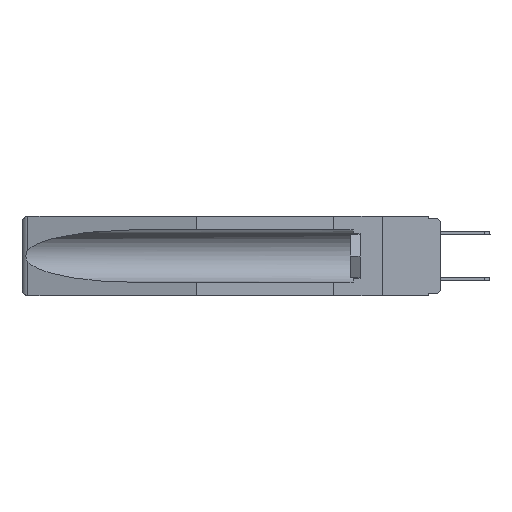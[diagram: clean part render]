
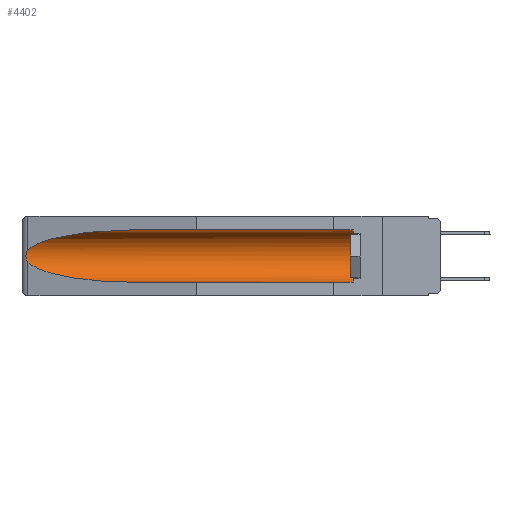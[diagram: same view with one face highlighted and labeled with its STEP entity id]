
A CAD part, left-side view. The second image highlights one B-rep face of the part: STEP entity #4402.
In plain terms, the highlighted cylindrical face has radius 2.857 mm (diameter 5.715 mm), a partial arc.
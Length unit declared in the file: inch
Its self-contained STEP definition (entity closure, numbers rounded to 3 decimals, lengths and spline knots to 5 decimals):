
#233 = CARTESIAN_POINT ( 'NONE',  ( 0.2675, 1.53308, -0.16763 ) ) ;
#564 = CARTESIAN_POINT ( 'NONE',  ( 0.21114, 1.30732, -0.059 ) ) ;
#1021 = CARTESIAN_POINT ( 'NONE',  ( 0.155, 1.07973, -0.284 ) ) ;
#1022 = ORIENTED_EDGE ( 'NONE', *, *, #17976, .T. ) ;
#1430 = LINE ( 'NONE', #1641, #16844 ) ;
#1641 = CARTESIAN_POINT ( 'NONE',  ( 0.155, -0.30754, -0.059 ) ) ;
#2132 = CARTESIAN_POINT ( 'NONE',  ( 0.155, 1.07973, -0.059 ) ) ;
#2237 = CARTESIAN_POINT ( 'NONE',  ( 0.25451, 1.48313, -0.09465 ) ) ;
#2512 = CARTESIAN_POINT ( 'NONE',  ( 0.155, 0.126, -0.059 ) ) ;
#2691 = FACE_OUTER_BOUND ( 'NONE', #11724, .T. ) ;
#2949 = CARTESIAN_POINT ( 'NONE',  ( 0.26597, 1.5296, -0.19026 ) ) ;
#3265 = CARTESIAN_POINT ( 'NONE',  ( 0.26537, 1.52718, -0.19328 ) ) ;
#3287 =( BOUNDED_CURVE ( )  B_SPLINE_CURVE ( 3, ( #2132, #564, #2237, #11764 ),
 .UNSPECIFIED., .F., .F. ) 
 B_SPLINE_CURVE_WITH_KNOTS ( ( 4, 4 ),
 ( 4.71239, 6.08839 ),
 .UNSPECIFIED. ) 
 CURVE ( )  GEOMETRIC_REPRESENTATION_ITEM ( )  RATIONAL_B_SPLINE_CURVE ( ( 1., 0.848, 0.848, 1. ) ) 
 REPRESENTATION_ITEM ( '' )  );
#4231 = VERTEX_POINT ( 'NONE', #16061 ) ;
#4356 = CARTESIAN_POINT ( 'NONE',  ( 0.25451, 1.48313, -0.24835 ) ) ;
#4402 = ADVANCED_FACE ( 'NONE', ( #2691 ), #16891, .F. ) ;
#4617 = CARTESIAN_POINT ( 'NONE',  ( 0.26655, 1.53094, -0.18657 ) ) ;
#4710 = CARTESIAN_POINT ( 'NONE',  ( 0.155, 1.07973, -0.284 ) ) ;
#4714 = CARTESIAN_POINT ( 'NONE',  ( 0.2673, 1.5327, -0.16383 ) ) ;
#5060 = ORIENTED_EDGE ( 'NONE', *, *, #8075, .T. ) ;
#5434 = ORIENTED_EDGE ( 'NONE', *, *, #13856, .T. ) ;
#5784 = CARTESIAN_POINT ( 'NONE',  ( 0.155, 0.126, -0.1715 ) ) ;
#6105 = VERTEX_POINT ( 'NONE', #10106 ) ;
#6352 = DIRECTION ( 'NONE',  ( 0., 1., 0. ) ) ;
#6430 = EDGE_CURVE ( 'NONE', #4231, #14896, #3287, .T. ) ;
#6797 = VERTEX_POINT ( 'NONE', #4710 ) ;
#7406 = DIRECTION ( 'NONE',  ( 0., 0., 1. ) ) ;
#8075 = EDGE_CURVE ( 'NONE', #14896, #6105, #18001, .T. ) ;
#8991 = CARTESIAN_POINT ( 'NONE',  ( 0.26537, 1.52718, -0.19328 ) ) ;
#9757 = CARTESIAN_POINT ( 'NONE',  ( 0.26537, 1.52718, -0.14972 ) ) ;
#9837 = ORIENTED_EDGE ( 'NONE', *, *, #15419, .F. ) ;
#10106 = CARTESIAN_POINT ( 'NONE',  ( 0.26537, 1.52718, -0.19328 ) ) ;
#10739 = CARTESIAN_POINT ( 'NONE',  ( 0.21114, 1.30732, -0.284 ) ) ;
#11294 = VERTEX_POINT ( 'NONE', #11916 ) ;
#11454 = CARTESIAN_POINT ( 'NONE',  ( 0.155, -0.30754, -0.284 ) ) ;
#11478 = VECTOR ( 'NONE', #11559, 39.37008 ) ;
#11559 = DIRECTION ( 'NONE',  ( 0., 1., 0. ) ) ;
#11724 = EDGE_LOOP ( 'NONE', ( #20489, #5060, #5434, #9837, #19543, #1022 ) ) ;
#11764 = CARTESIAN_POINT ( 'NONE',  ( 0.26537, 1.52718, -0.14972 ) ) ;
#11916 = CARTESIAN_POINT ( 'NONE',  ( 0.155, 0.126, -0.284 ) ) ;
#12259 = AXIS2_PLACEMENT_3D ( 'NONE', #17091, #15426, #7406 ) ;
#13856 = EDGE_CURVE ( 'NONE', #6105, #6797, #15308, .T. ) ;
#14105 = CIRCLE ( 'NONE', #15117, 0.1125 ) ;
#14318 = EDGE_CURVE ( 'NONE', #11294, #16727, #14105, .T. ) ;
#14367 = LINE ( 'NONE', #11454, #11478 ) ;
#14896 = VERTEX_POINT ( 'NONE', #16936 ) ;
#15117 = AXIS2_PLACEMENT_3D ( 'NONE', #5784, #18815, #20287 ) ;
#15308 =( BOUNDED_CURVE ( )  B_SPLINE_CURVE ( 3, ( #8991, #4356, #10739, #1021 ),
 .UNSPECIFIED., .F., .F. ) 
 B_SPLINE_CURVE_WITH_KNOTS ( ( 4, 4 ),
 ( 0.1948, 1.5708 ),
 .UNSPECIFIED. ) 
 CURVE ( )  GEOMETRIC_REPRESENTATION_ITEM ( )  RATIONAL_B_SPLINE_CURVE ( ( 1., 0.848, 0.848, 1. ) ) 
 REPRESENTATION_ITEM ( '' )  );
#15419 = EDGE_CURVE ( 'NONE', #11294, #6797, #14367, .T. ) ;
#15426 = DIRECTION ( 'NONE',  ( 0., 1., 0. ) ) ;
#15792 = CARTESIAN_POINT ( 'NONE',  ( 0.2673, 1.53269, -0.17917 ) ) ;
#16061 = CARTESIAN_POINT ( 'NONE',  ( 0.155, 1.07973, -0.059 ) ) ;
#16727 = VERTEX_POINT ( 'NONE', #2512 ) ;
#16844 = VECTOR ( 'NONE', #6352, 39.37008 ) ;
#16891 = CYLINDRICAL_SURFACE ( 'NONE', #12259, 0.1125 ) ;
#16936 = CARTESIAN_POINT ( 'NONE',  ( 0.26537, 1.52718, -0.14972 ) ) ;
#17091 = CARTESIAN_POINT ( 'NONE',  ( 0.155, -0.30754, -0.1715 ) ) ;
#17252 = CARTESIAN_POINT ( 'NONE',  ( 0.2675, 1.53308, -0.17534 ) ) ;
#17357 = CARTESIAN_POINT ( 'NONE',  ( 0.26654, 1.53092, -0.15636 ) ) ;
#17976 = EDGE_CURVE ( 'NONE', #16727, #4231, #1430, .T. ) ;
#18001 = B_SPLINE_CURVE_WITH_KNOTS ( 'NONE', 3,
 ( #9757, #20593, #17357, #4714, #233, #17252, #15792, #4617, #2949, #3265 ),
 .UNSPECIFIED., .F., .F.,
 ( 4, 2, 2, 2, 4 ),
 ( 0., 0.00029, 0.00058, 0.00087, 0.00117 ),
 .UNSPECIFIED. ) ;
#18815 = DIRECTION ( 'NONE',  ( 0., -1., 0. ) ) ;
#19543 = ORIENTED_EDGE ( 'NONE', *, *, #14318, .T. ) ;
#20287 = DIRECTION ( 'NONE',  ( 0., 0., 1. ) ) ;
#20489 = ORIENTED_EDGE ( 'NONE', *, *, #6430, .T. ) ;
#20593 = CARTESIAN_POINT ( 'NONE',  ( 0.26597, 1.52961, -0.15275 ) ) ;
